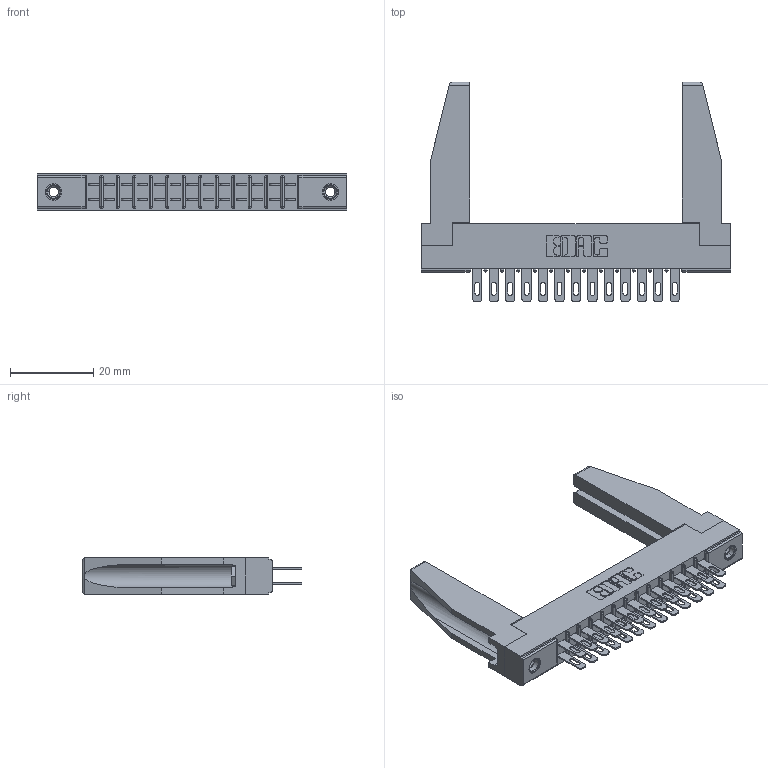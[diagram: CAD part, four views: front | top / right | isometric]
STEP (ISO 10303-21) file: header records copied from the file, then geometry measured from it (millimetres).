
FILE_DESCRIPTION (( 'STEP AP203' ), '1' );
FILE_NAME ('355-026-500-578.STEP', '2019-09-11T05:22:06', ( '' ), ( '' ), 'SwSTEP 2.0', 'SolidWorks 2016', '' );
FILE_SCHEMA (( 'CONFIG_CONTROL_DESIGN' ));
Length unit declared in the file: inch
Products named in the file (5): 305 Part_.156 Dia; 355-026-500-578; 345-250-001_345-250-001-102; 305-290-001_500; 307-220-078
Assembly tree (31 placements, depth 2):
  355-026-500-578
    305 Part_.156 Dia
    305-290-001_500  x26
    345-250-001_345-250-001-102  x2
    307-220-078  x2
Bounding box: 74.52 x 52.88 x 8.71 mm (x, y, z)
Volume: 8574.9 mm3; surface area: 12825 mm2
Topology: 31 solids, 31 shells, 1546 faces, 4377 edges, 2838 vertices
Faces by surface type: plane 880, cylinder 598, sphere 52, cone 12, torus 4
Entity records: 20067 total; most frequent: CARTESIAN_POINT 3327, ORIENTED_EDGE 3256, DIRECTION 3202, EDGE_CURVE 1628, LINE 1280, VECTOR 1280, VERTEX_POINT 1044, AXIS2_PLACEMENT_3D 961
